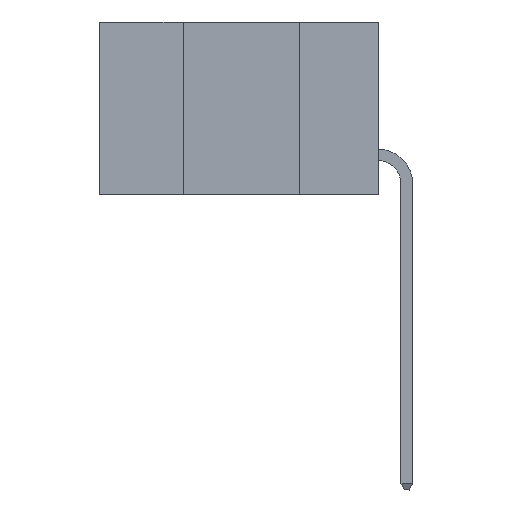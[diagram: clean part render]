
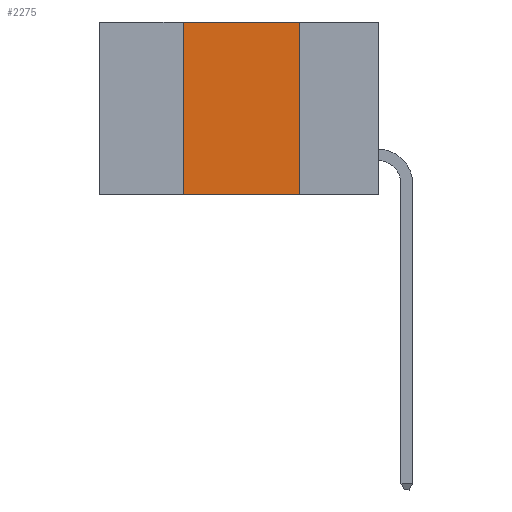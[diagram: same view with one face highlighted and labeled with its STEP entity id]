
A CAD part, left-side view. The second image highlights one B-rep face of the part: STEP entity #2275.
In plain terms, the highlighted planar face has unit normal (-1, 0, 0).
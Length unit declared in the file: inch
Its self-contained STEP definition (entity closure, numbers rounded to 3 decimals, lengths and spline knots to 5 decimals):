
#162 = DIRECTION ( 'NONE',  ( 0., 0., 1. ) ) ;
#257 = CARTESIAN_POINT ( 'NONE',  ( 0., 0.6, 0. ) ) ;
#826 = VECTOR ( 'NONE', #7724, 39.37008 ) ;
#1117 = DIRECTION ( 'NONE',  ( 0., 0., -1. ) ) ;
#1463 = ORIENTED_EDGE ( 'NONE', *, *, #8558, .T. ) ;
#1832 = CARTESIAN_POINT ( 'NONE',  ( 0., 0.42, 0. ) ) ;
#1927 = DIRECTION ( 'NONE',  ( 0., -1., 0. ) ) ;
#2275 = ADVANCED_FACE ( 'NONE', ( #10130 ), #4385, .F. ) ;
#2341 = EDGE_CURVE ( 'NONE', #4822, #4941, #10205, .T. ) ;
#2433 = EDGE_LOOP ( 'NONE', ( #4197, #9064, #6031, #1463 ) ) ;
#2687 = LINE ( 'NONE', #6061, #7872 ) ;
#2925 = VECTOR ( 'NONE', #162, 39.37008 ) ;
#3563 = DIRECTION ( 'NONE',  ( 1., 0., 0. ) ) ;
#3761 = CARTESIAN_POINT ( 'NONE',  ( 0., 0.17, -0.37 ) ) ;
#3986 = EDGE_CURVE ( 'NONE', #10364, #5407, #8417, .T. ) ;
#4115 = AXIS2_PLACEMENT_3D ( 'NONE', #257, #3563, #1117 ) ;
#4197 = ORIENTED_EDGE ( 'NONE', *, *, #2341, .F. ) ;
#4290 = CARTESIAN_POINT ( 'NONE',  ( 0., 0.42, -0.37 ) ) ;
#4385 = PLANE ( 'NONE',  #4115 ) ;
#4731 = VECTOR ( 'NONE', #7594, 39.37008 ) ;
#4822 = VERTEX_POINT ( 'NONE', #9628 ) ;
#4941 = VERTEX_POINT ( 'NONE', #7290 ) ;
#5154 = LINE ( 'NONE', #8570, #4731 ) ;
#5407 = VERTEX_POINT ( 'NONE', #1832 ) ;
#5501 = EDGE_CURVE ( 'NONE', #5407, #4822, #5154, .T. ) ;
#6031 = ORIENTED_EDGE ( 'NONE', *, *, #3986, .F. ) ;
#6061 = CARTESIAN_POINT ( 'NONE',  ( 0., 0.6, -0.37 ) ) ;
#7290 = CARTESIAN_POINT ( 'NONE',  ( 0., 0.17, -0.37 ) ) ;
#7594 = DIRECTION ( 'NONE',  ( 0., -1., 0. ) ) ;
#7724 = DIRECTION ( 'NONE',  ( 0., 0., -1. ) ) ;
#7872 = VECTOR ( 'NONE', #1927, 39.37008 ) ;
#8417 = LINE ( 'NONE', #4290, #2925 ) ;
#8558 = EDGE_CURVE ( 'NONE', #10364, #4941, #2687, .T. ) ;
#8570 = CARTESIAN_POINT ( 'NONE',  ( 0., 0.6, 0. ) ) ;
#9064 = ORIENTED_EDGE ( 'NONE', *, *, #5501, .F. ) ;
#9343 = CARTESIAN_POINT ( 'NONE',  ( 0., 0.42, -0.37 ) ) ;
#9628 = CARTESIAN_POINT ( 'NONE',  ( 0., 0.17, 0. ) ) ;
#10130 = FACE_OUTER_BOUND ( 'NONE', #2433, .T. ) ;
#10205 = LINE ( 'NONE', #3761, #826 ) ;
#10364 = VERTEX_POINT ( 'NONE', #9343 ) ;
